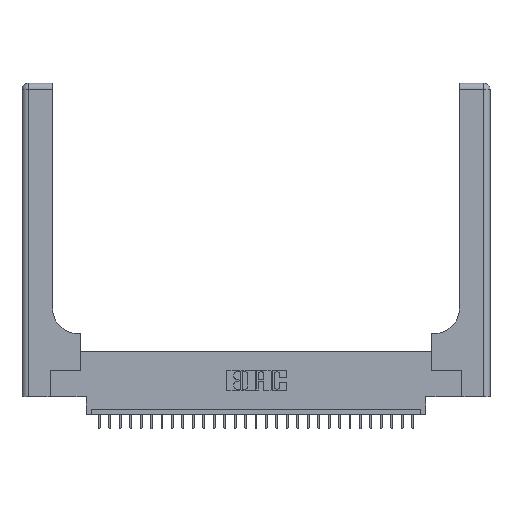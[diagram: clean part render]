
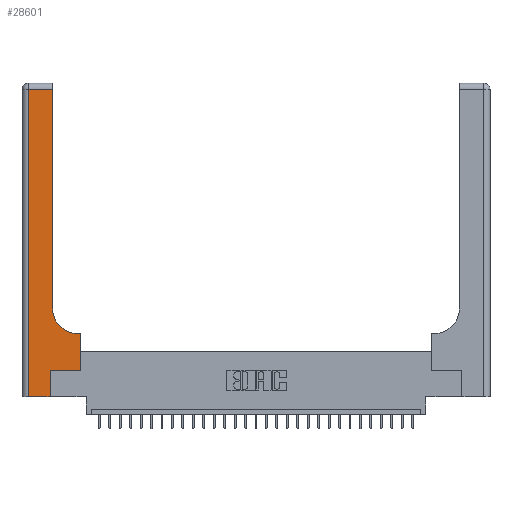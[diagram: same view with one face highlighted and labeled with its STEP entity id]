
A CAD part, top view. The second image highlights one B-rep face of the part: STEP entity #28601.
In plain terms, the highlighted planar face has unit normal (0, 0, 1).
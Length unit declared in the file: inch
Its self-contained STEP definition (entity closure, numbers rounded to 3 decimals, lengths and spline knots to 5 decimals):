
#997 = VECTOR ( 'NONE', #12412, 39.37008 ) ;
#1032 = CARTESIAN_POINT ( 'NONE',  ( 0.5585, 0.25, 0.37 ) ) ;
#1273 = VECTOR ( 'NONE', #24938, 39.37008 ) ;
#1282 = EDGE_CURVE ( 'NONE', #20454, #28331, #23558, .T. ) ;
#2239 = ORIENTED_EDGE ( 'NONE', *, *, #1282, .T. ) ;
#2675 = VECTOR ( 'NONE', #15593, 39.37008 ) ;
#3376 = CARTESIAN_POINT ( 'NONE',  ( 0.5585, 0.6, 0.37 ) ) ;
#4885 = LINE ( 'NONE', #14201, #9288 ) ;
#5516 = DIRECTION ( 'NONE',  ( 0., 0., -1. ) ) ;
#6038 = CARTESIAN_POINT ( 'NONE',  ( 0.269, 0., 0.37 ) ) ;
#6122 = DIRECTION ( 'NONE',  ( 0., 1., 0. ) ) ;
#6194 = EDGE_CURVE ( 'NONE', #28331, #21216, #29044, .T. ) ;
#6244 = VERTEX_POINT ( 'NONE', #3376 ) ;
#6290 = LINE ( 'NONE', #27225, #2675 ) ;
#6681 = DIRECTION ( 'NONE',  ( 0., 0., -1. ) ) ;
#6941 = LINE ( 'NONE', #16243, #21167 ) ;
#7932 = LINE ( 'NONE', #19097, #25787 ) ;
#8224 = CARTESIAN_POINT ( 'NONE',  ( 0.5415, 0.6, 0.37 ) ) ;
#8296 = CARTESIAN_POINT ( 'NONE',  ( 0.2915, 2.94, 0.37 ) ) ;
#8557 = LINE ( 'NONE', #13000, #29681 ) ;
#9132 = CARTESIAN_POINT ( 'NONE',  ( 0., 2.94, 0.37 ) ) ;
#9208 = EDGE_CURVE ( 'NONE', #21216, #9836, #27624, .T. ) ;
#9288 = VECTOR ( 'NONE', #16339, 39.37008 ) ;
#9836 = VERTEX_POINT ( 'NONE', #11046 ) ;
#10282 = CARTESIAN_POINT ( 'NONE',  ( 0.2915, 0.85, 0.37 ) ) ;
#10758 = ORIENTED_EDGE ( 'NONE', *, *, #6194, .T. ) ;
#11046 = CARTESIAN_POINT ( 'NONE',  ( 0.06, 2.94, 0.37 ) ) ;
#11263 = CARTESIAN_POINT ( 'NONE',  ( 0.5415, 0.85, 0.37 ) ) ;
#12110 = CARTESIAN_POINT ( 'NONE',  ( 0.2915, 3., 0.37 ) ) ;
#12269 = ORIENTED_EDGE ( 'NONE', *, *, #25103, .T. ) ;
#12412 = DIRECTION ( 'NONE',  ( 0., 1., 0. ) ) ;
#13000 = CARTESIAN_POINT ( 'NONE',  ( 0.269, 0., 0.37 ) ) ;
#14201 = CARTESIAN_POINT ( 'NONE',  ( 0.2915, 0.6, 0.37 ) ) ;
#14536 = PLANE ( 'NONE',  #30108 ) ;
#15593 = DIRECTION ( 'NONE',  ( 0., -1., 0. ) ) ;
#16243 = CARTESIAN_POINT ( 'NONE',  ( 0.5585, 0.25, 0.37 ) ) ;
#16339 = DIRECTION ( 'NONE',  ( -1., 0., 0. ) ) ;
#16471 = EDGE_CURVE ( 'NONE', #29545, #29705, #8557, .T. ) ;
#16790 = EDGE_CURVE ( 'NONE', #16920, #29545, #7932, .T. ) ;
#16920 = VERTEX_POINT ( 'NONE', #25605 ) ;
#17462 = VECTOR ( 'NONE', #22887, 39.37008 ) ;
#17470 = ORIENTED_EDGE ( 'NONE', *, *, #26049, .T. ) ;
#17840 = DIRECTION ( 'NONE',  ( 1., 0., 0. ) ) ;
#18436 = ORIENTED_EDGE ( 'NONE', *, *, #16471, .T. ) ;
#18992 = EDGE_CURVE ( 'NONE', #6244, #20454, #4885, .T. ) ;
#19097 = CARTESIAN_POINT ( 'NONE',  ( 0., 0., 0.37 ) ) ;
#19143 = CARTESIAN_POINT ( 'NONE',  ( 0.269, 0.25, 0.37 ) ) ;
#19974 = ORIENTED_EDGE ( 'NONE', *, *, #9208, .T. ) ;
#20454 = VERTEX_POINT ( 'NONE', #8224 ) ;
#21167 = VECTOR ( 'NONE', #21748, 39.37008 ) ;
#21216 = VERTEX_POINT ( 'NONE', #8296 ) ;
#21224 = EDGE_LOOP ( 'NONE', ( #10758, #19974, #17470, #23907, #18436, #29847, #12269, #23140, #2239 ) ) ;
#21748 = DIRECTION ( 'NONE',  ( 0., 1., 0. ) ) ;
#22487 = LINE ( 'NONE', #27385, #1273 ) ;
#22887 = DIRECTION ( 'NONE',  ( -1., 0., 0. ) ) ;
#23140 = ORIENTED_EDGE ( 'NONE', *, *, #18992, .T. ) ;
#23558 = CIRCLE ( 'NONE', #27462, 0.25 ) ;
#23865 = CARTESIAN_POINT ( 'NONE',  ( 0., 3., 0.37 ) ) ;
#23907 = ORIENTED_EDGE ( 'NONE', *, *, #16790, .T. ) ;
#24450 = DIRECTION ( 'NONE',  ( -1., 0., 0. ) ) ;
#24938 = DIRECTION ( 'NONE',  ( 1., 0., 0. ) ) ;
#25103 = EDGE_CURVE ( 'NONE', #25504, #6244, #6941, .T. ) ;
#25504 = VERTEX_POINT ( 'NONE', #1032 ) ;
#25605 = CARTESIAN_POINT ( 'NONE',  ( 0.06, 0., 0.37 ) ) ;
#25787 = VECTOR ( 'NONE', #28865, 39.37008 ) ;
#26049 = EDGE_CURVE ( 'NONE', #9836, #16920, #6290, .T. ) ;
#27225 = CARTESIAN_POINT ( 'NONE',  ( 0.06, 3., 0.37 ) ) ;
#27385 = CARTESIAN_POINT ( 'NONE',  ( 0.269, 0.25, 0.37 ) ) ;
#27462 = AXIS2_PLACEMENT_3D ( 'NONE', #11263, #6681, #17840 ) ;
#27624 = LINE ( 'NONE', #9132, #17462 ) ;
#28331 = VERTEX_POINT ( 'NONE', #10282 ) ;
#28376 = EDGE_CURVE ( 'NONE', #29705, #25504, #22487, .T. ) ;
#28592 = FACE_OUTER_BOUND ( 'NONE', #21224, .T. ) ;
#28601 = ADVANCED_FACE ( 'NONE', ( #28592 ), #14536, .F. ) ;
#28865 = DIRECTION ( 'NONE',  ( 1., 0., 0. ) ) ;
#29044 = LINE ( 'NONE', #12110, #997 ) ;
#29545 = VERTEX_POINT ( 'NONE', #6038 ) ;
#29681 = VECTOR ( 'NONE', #6122, 39.37008 ) ;
#29705 = VERTEX_POINT ( 'NONE', #19143 ) ;
#29847 = ORIENTED_EDGE ( 'NONE', *, *, #28376, .T. ) ;
#30108 = AXIS2_PLACEMENT_3D ( 'NONE', #23865, #5516, #24450 ) ;
